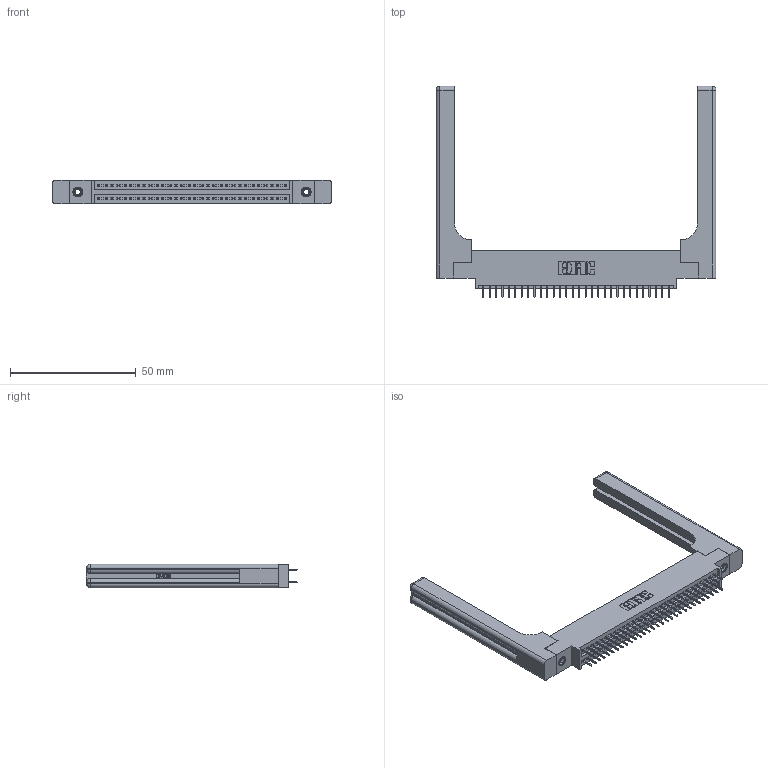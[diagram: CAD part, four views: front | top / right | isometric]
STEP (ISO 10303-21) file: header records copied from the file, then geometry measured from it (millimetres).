
FILE_DESCRIPTION (( 'STEP AP203' ), '1' );
FILE_NAME ('395-060-525-858.STEP', '2020-09-24T20:55:05', ( '' ), ( '' ), 'SwSTEP 2.0', 'SolidWorks 2020', '' );
FILE_SCHEMA (( 'CONFIG_CONTROL_DESIGN' ));
Length unit declared in the file: inch
Products named in the file (5): 345-292-001_345-293-125; 345-220-058_345-220-058; 345 Part_0.170 Offset - 0.156 Dia-TH; 345-250-001_345-250-001-102; 395-060-525-858
Assembly tree (65 placements, depth 2):
  395-060-525-858
    345 Part_0.170 Offset - 0.156 Dia-TH
    345-292-001_345-293-125  x60
    345-250-001_345-250-001-102  x2
    345-220-058_345-220-058  x2
Bounding box: 111.23 x 84 x 9.4 mm (x, y, z)
Volume: 18956.2 mm3; surface area: 20165.2 mm2
Topology: 65 solids, 65 shells, 3626 faces, 10199 edges, 6538 vertices
Faces by surface type: plane 2572, cylinder 994, bspline 36, cone 12, sphere 8, torus 4
Entity records: 30542 total; most frequent: CARTESIAN_POINT 6125, ORIENTED_EDGE 4856, DIRECTION 4348, EDGE_CURVE 2428, LINE 2088, VECTOR 2088, VERTEX_POINT 1606, AXIS2_PLACEMENT_3D 1130
